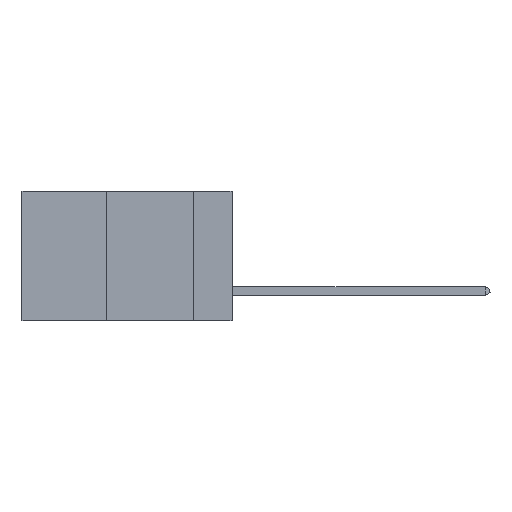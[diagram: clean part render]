
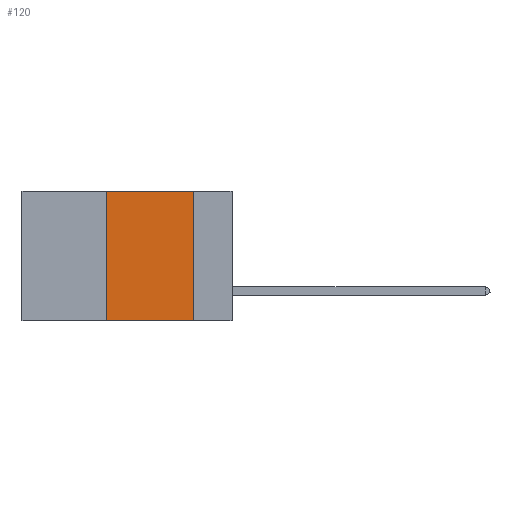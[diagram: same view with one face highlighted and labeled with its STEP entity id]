
A CAD part, left-side view. The second image highlights one B-rep face of the part: STEP entity #120.
In plain terms, the highlighted planar face has unit normal (-1, 0, 0).
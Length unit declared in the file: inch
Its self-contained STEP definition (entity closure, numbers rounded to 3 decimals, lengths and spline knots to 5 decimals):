
#120 = ADVANCED_FACE ( 'NONE', ( #4932 ), #1749, .F. ) ;
#382 = LINE ( 'NONE', #8746, #5112 ) ;
#627 = ORIENTED_EDGE ( 'NONE', *, *, #9238, .F. ) ;
#849 = VERTEX_POINT ( 'NONE', #6980 ) ;
#953 = VERTEX_POINT ( 'NONE', #12568 ) ;
#1454 = DIRECTION ( 'NONE',  ( 0., -1., 0. ) ) ;
#1484 = ORIENTED_EDGE ( 'NONE', *, *, #9324, .F. ) ;
#1749 = PLANE ( 'NONE',  #2261 ) ;
#2261 = AXIS2_PLACEMENT_3D ( 'NONE', #12264, #11063, #11143 ) ;
#2387 = ORIENTED_EDGE ( 'NONE', *, *, #10576, .T. ) ;
#3004 = EDGE_LOOP ( 'NONE', ( #3297, #1484, #627, #2387 ) ) ;
#3297 = ORIENTED_EDGE ( 'NONE', *, *, #10139, .F. ) ;
#3326 = CARTESIAN_POINT ( 'NONE',  ( 0., 0.36, -0.37 ) ) ;
#4096 = DIRECTION ( 'NONE',  ( 0., 0., 1. ) ) ;
#4454 = DIRECTION ( 'NONE',  ( 0., 0., -1. ) ) ;
#4932 = FACE_OUTER_BOUND ( 'NONE', #3004, .T. ) ;
#5112 = VECTOR ( 'NONE', #1454, 39.37008 ) ;
#5435 = LINE ( 'NONE', #11743, #7897 ) ;
#6423 = VERTEX_POINT ( 'NONE', #3326 ) ;
#6745 = VECTOR ( 'NONE', #4454, 39.37008 ) ;
#6980 = CARTESIAN_POINT ( 'NONE',  ( 0., 0.11, -0.37 ) ) ;
#6985 = DIRECTION ( 'NONE',  ( 0., -1., 0. ) ) ;
#7403 = LINE ( 'NONE', #10305, #6745 ) ;
#7543 = VECTOR ( 'NONE', #6985, 39.37008 ) ;
#7897 = VECTOR ( 'NONE', #4096, 39.37008 ) ;
#8746 = CARTESIAN_POINT ( 'NONE',  ( 0., 0.6, 0. ) ) ;
#9238 = EDGE_CURVE ( 'NONE', #6423, #11603, #5435, .T. ) ;
#9324 = EDGE_CURVE ( 'NONE', #11603, #953, #382, .T. ) ;
#10139 = EDGE_CURVE ( 'NONE', #953, #849, #7403, .T. ) ;
#10305 = CARTESIAN_POINT ( 'NONE',  ( 0., 0.11, 0. ) ) ;
#10576 = EDGE_CURVE ( 'NONE', #6423, #849, #12784, .T. ) ;
#10994 = CARTESIAN_POINT ( 'NONE',  ( 0., 0.36, 0. ) ) ;
#11063 = DIRECTION ( 'NONE',  ( 1., 0., 0. ) ) ;
#11143 = DIRECTION ( 'NONE',  ( 0., 0., -1. ) ) ;
#11603 = VERTEX_POINT ( 'NONE', #10994 ) ;
#11743 = CARTESIAN_POINT ( 'NONE',  ( 0., 0.36, 0. ) ) ;
#12264 = CARTESIAN_POINT ( 'NONE',  ( 0., 0.6, 0. ) ) ;
#12568 = CARTESIAN_POINT ( 'NONE',  ( 0., 0.11, 0. ) ) ;
#12784 = LINE ( 'NONE', #13272, #7543 ) ;
#13272 = CARTESIAN_POINT ( 'NONE',  ( 0., 0.6, -0.37 ) ) ;
